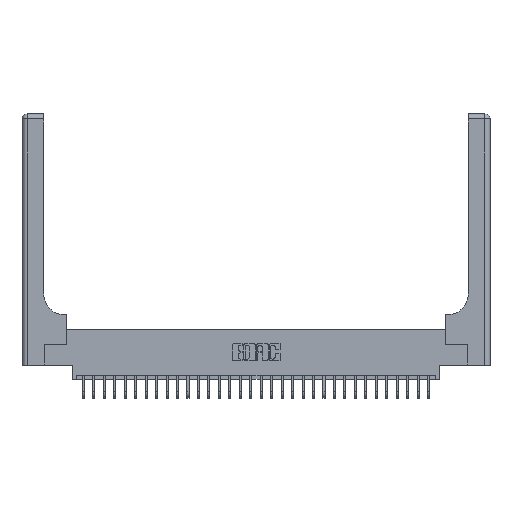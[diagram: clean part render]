
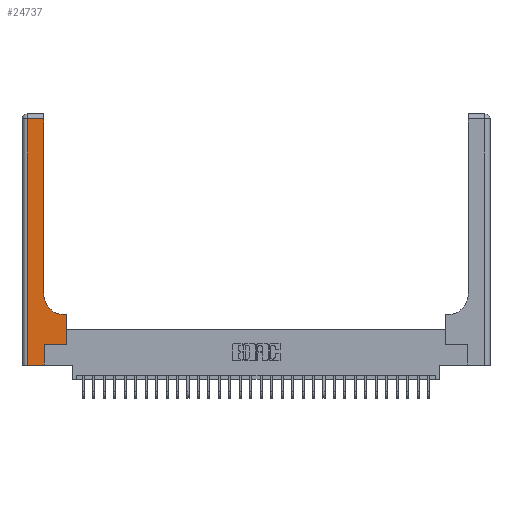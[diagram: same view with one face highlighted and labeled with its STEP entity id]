
A CAD part, top view. The second image highlights one B-rep face of the part: STEP entity #24737.
In plain terms, the highlighted planar face has unit normal (0, 0, 1).
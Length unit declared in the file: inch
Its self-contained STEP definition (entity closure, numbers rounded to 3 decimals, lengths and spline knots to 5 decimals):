
#1024 = CARTESIAN_POINT ( 'NONE',  ( 0., 3., 0.37 ) ) ;
#1026 = CARTESIAN_POINT ( 'NONE',  ( 0.26, 0.6, 0.37 ) ) ;
#1550 = ORIENTED_EDGE ( 'NONE', *, *, #7986, .T. ) ;
#1820 = CIRCLE ( 'NONE', #29226, 0.25 ) ;
#2073 = ORIENTED_EDGE ( 'NONE', *, *, #11300, .T. ) ;
#2116 = VERTEX_POINT ( 'NONE', #9971 ) ;
#2377 = EDGE_CURVE ( 'NONE', #2116, #2469, #1820, .T. ) ;
#2469 = VERTEX_POINT ( 'NONE', #28768 ) ;
#2849 = CARTESIAN_POINT ( 'NONE',  ( 0.06, 0., 0.37 ) ) ;
#2954 = ORIENTED_EDGE ( 'NONE', *, *, #7190, .T. ) ;
#3031 = DIRECTION ( 'NONE',  ( -1., 0., 0. ) ) ;
#4007 = ORIENTED_EDGE ( 'NONE', *, *, #29750, .T. ) ;
#5016 = ORIENTED_EDGE ( 'NONE', *, *, #14675, .T. ) ;
#6787 = CARTESIAN_POINT ( 'NONE',  ( 0.51, 0.85, 0.37 ) ) ;
#7190 = EDGE_CURVE ( 'NONE', #15130, #13179, #7857, .T. ) ;
#7262 = CARTESIAN_POINT ( 'NONE',  ( 0.265, 0.25, 0.37 ) ) ;
#7288 = AXIS2_PLACEMENT_3D ( 'NONE', #1024, #10239, #3031 ) ;
#7857 = LINE ( 'NONE', #16922, #9146 ) ;
#7986 = EDGE_CURVE ( 'NONE', #13179, #24563, #30118, .T. ) ;
#8049 = VECTOR ( 'NONE', #20097, 39.37008 ) ;
#8847 = CARTESIAN_POINT ( 'NONE',  ( 0.528, 0.25, 0.37 ) ) ;
#8972 = DIRECTION ( 'NONE',  ( 0., 1., 0. ) ) ;
#9146 = VECTOR ( 'NONE', #14570, 39.37008 ) ;
#9428 = DIRECTION ( 'NONE',  ( 0., 0., -1. ) ) ;
#9685 = LINE ( 'NONE', #30336, #28532 ) ;
#9941 = VECTOR ( 'NONE', #12131, 39.37008 ) ;
#9971 = CARTESIAN_POINT ( 'NONE',  ( 0.51, 0.6, 0.37 ) ) ;
#10239 = DIRECTION ( 'NONE',  ( 0., 0., -1. ) ) ;
#10994 = EDGE_CURVE ( 'NONE', #22637, #25151, #23810, .T. ) ;
#10999 = CARTESIAN_POINT ( 'NONE',  ( 0.265, 0.25, 0.37 ) ) ;
#11006 = EDGE_LOOP ( 'NONE', ( #15242, #24177, #2073, #2954, #1550, #4007, #14782, #5016, #18011 ) ) ;
#11207 = CARTESIAN_POINT ( 'NONE',  ( 0.265, 0., 0.37 ) ) ;
#11300 = EDGE_CURVE ( 'NONE', #25151, #15130, #18671, .T. ) ;
#12131 = DIRECTION ( 'NONE',  ( 0., 1., 0. ) ) ;
#12237 = CARTESIAN_POINT ( 'NONE',  ( 0.26, 2.94, 0.37 ) ) ;
#12653 = VECTOR ( 'NONE', #29968, 39.37008 ) ;
#13179 = VERTEX_POINT ( 'NONE', #11207 ) ;
#13189 = LINE ( 'NONE', #1026, #8049 ) ;
#14454 = LINE ( 'NONE', #23968, #9941 ) ;
#14570 = DIRECTION ( 'NONE',  ( 1., 0., 0. ) ) ;
#14675 = EDGE_CURVE ( 'NONE', #18597, #2116, #13189, .T. ) ;
#14782 = ORIENTED_EDGE ( 'NONE', *, *, #29030, .T. ) ;
#15130 = VERTEX_POINT ( 'NONE', #2849 ) ;
#15242 = ORIENTED_EDGE ( 'NONE', *, *, #25168, .T. ) ;
#15521 = LINE ( 'NONE', #10999, #28910 ) ;
#15753 = VECTOR ( 'NONE', #30795, 39.37008 ) ;
#16205 = CARTESIAN_POINT ( 'NONE',  ( 0., 2.94, 0.37 ) ) ;
#16922 = CARTESIAN_POINT ( 'NONE',  ( 0., 0., 0.37 ) ) ;
#18011 = ORIENTED_EDGE ( 'NONE', *, *, #2377, .T. ) ;
#18597 = VERTEX_POINT ( 'NONE', #26595 ) ;
#18671 = LINE ( 'NONE', #30351, #15753 ) ;
#20097 = DIRECTION ( 'NONE',  ( -1., 0., 0. ) ) ;
#20532 = DIRECTION ( 'NONE',  ( 1., 0., 0. ) ) ;
#21627 = PLANE ( 'NONE',  #7288 ) ;
#22637 = VERTEX_POINT ( 'NONE', #12237 ) ;
#22939 = CARTESIAN_POINT ( 'NONE',  ( 0.265, 0., 0.37 ) ) ;
#23810 = LINE ( 'NONE', #16205, #24702 ) ;
#23950 = FACE_OUTER_BOUND ( 'NONE', #11006, .T. ) ;
#23968 = CARTESIAN_POINT ( 'NONE',  ( 0.528, 0.25, 0.37 ) ) ;
#24177 = ORIENTED_EDGE ( 'NONE', *, *, #10994, .T. ) ;
#24563 = VERTEX_POINT ( 'NONE', #7262 ) ;
#24702 = VECTOR ( 'NONE', #28670, 39.37008 ) ;
#24737 = ADVANCED_FACE ( 'NONE', ( #23950 ), #21627, .F. ) ;
#25151 = VERTEX_POINT ( 'NONE', #26383 ) ;
#25168 = EDGE_CURVE ( 'NONE', #2469, #22637, #9685, .T. ) ;
#26383 = CARTESIAN_POINT ( 'NONE',  ( 0.06, 2.94, 0.37 ) ) ;
#26595 = CARTESIAN_POINT ( 'NONE',  ( 0.528, 0.6, 0.37 ) ) ;
#28322 = DIRECTION ( 'NONE',  ( 1., 0., 0. ) ) ;
#28532 = VECTOR ( 'NONE', #8972, 39.37008 ) ;
#28670 = DIRECTION ( 'NONE',  ( -1., 0., 0. ) ) ;
#28768 = CARTESIAN_POINT ( 'NONE',  ( 0.26, 0.85, 0.37 ) ) ;
#28910 = VECTOR ( 'NONE', #20532, 39.37008 ) ;
#29030 = EDGE_CURVE ( 'NONE', #29294, #18597, #14454, .T. ) ;
#29226 = AXIS2_PLACEMENT_3D ( 'NONE', #6787, #9428, #28322 ) ;
#29294 = VERTEX_POINT ( 'NONE', #8847 ) ;
#29750 = EDGE_CURVE ( 'NONE', #24563, #29294, #15521, .T. ) ;
#29968 = DIRECTION ( 'NONE',  ( 0., 1., 0. ) ) ;
#30118 = LINE ( 'NONE', #22939, #12653 ) ;
#30336 = CARTESIAN_POINT ( 'NONE',  ( 0.26, 3., 0.37 ) ) ;
#30351 = CARTESIAN_POINT ( 'NONE',  ( 0.06, 3., 0.37 ) ) ;
#30795 = DIRECTION ( 'NONE',  ( 0., -1., 0. ) ) ;
